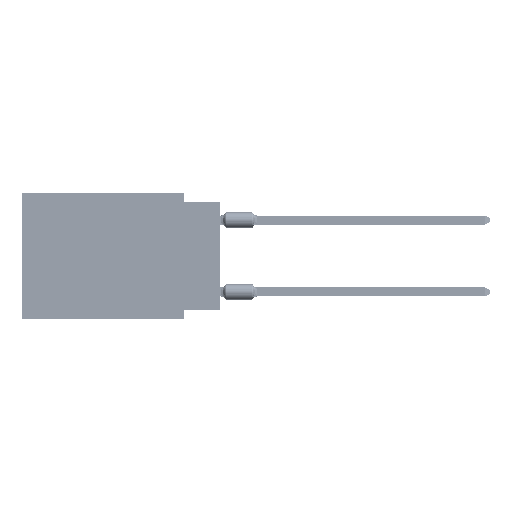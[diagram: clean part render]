
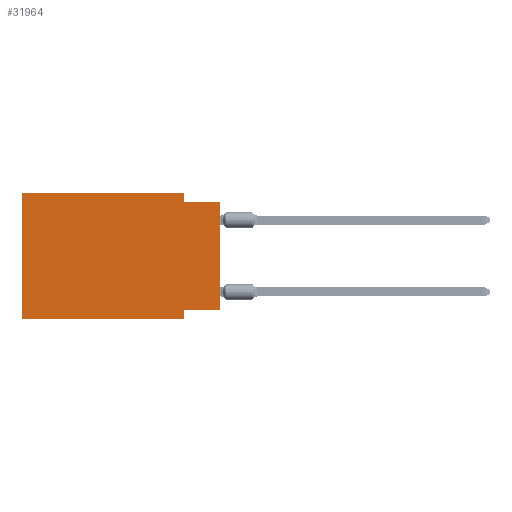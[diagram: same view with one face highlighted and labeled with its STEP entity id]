
A CAD part, left-side view. The second image highlights one B-rep face of the part: STEP entity #31964.
In plain terms, the highlighted planar face has unit normal (-1, 0, 0).
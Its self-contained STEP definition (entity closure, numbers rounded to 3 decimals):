
#1317 = ORIENTED_EDGE ( 'NONE', *, *, #56635, .F. ) ;
#4426 = EDGE_CURVE ( 'NONE', #86143, #73094, #27593, .T. ) ;
#5830 = CARTESIAN_POINT ( 'NONE',  ( 0., 13.97, -8.89 ) ) ;
#7325 = VECTOR ( 'NONE', #56872, 1000. ) ;
#10690 = VERTEX_POINT ( 'NONE', #80825 ) ;
#12012 = ORIENTED_EDGE ( 'NONE', *, *, #41503, .T. ) ;
#13321 = CARTESIAN_POINT ( 'NONE',  ( 0., 0., -8.255 ) ) ;
#13442 = DIRECTION ( 'NONE',  ( 0., 0., -1. ) ) ;
#14587 = CARTESIAN_POINT ( 'NONE',  ( 0., 13.97, 0. ) ) ;
#18264 = EDGE_LOOP ( 'NONE', ( #12012, #1317, #19668, #59747, #22438, #51683, #84203, #18834 ) ) ;
#18834 = ORIENTED_EDGE ( 'NONE', *, *, #32896, .F. ) ;
#19668 = ORIENTED_EDGE ( 'NONE', *, *, #21820, .F. ) ;
#20445 = CARTESIAN_POINT ( 'NONE',  ( 0., 13.97, 0. ) ) ;
#21051 = VERTEX_POINT ( 'NONE', #76989 ) ;
#21820 = EDGE_CURVE ( 'NONE', #10690, #73108, #37596, .T. ) ;
#22028 = DIRECTION ( 'NONE',  ( 0., 0., 1. ) ) ;
#22196 = CARTESIAN_POINT ( 'NONE',  ( 0., 2.54, 0. ) ) ;
#22438 = ORIENTED_EDGE ( 'NONE', *, *, #80332, .F. ) ;
#23707 = CARTESIAN_POINT ( 'NONE',  ( 0., 13.97, -8.89 ) ) ;
#24312 = AXIS2_PLACEMENT_3D ( 'NONE', #20445, #77865, #13442 ) ;
#27593 = LINE ( 'NONE', #49036, #48803 ) ;
#28555 = CARTESIAN_POINT ( 'NONE',  ( 0., 0., 0. ) ) ;
#29881 = EDGE_CURVE ( 'NONE', #78756, #73094, #51234, .T. ) ;
#31964 = ADVANCED_FACE ( 'NONE', ( #56815 ), #84426, .F. ) ;
#32896 = EDGE_CURVE ( 'NONE', #46298, #86143, #88183, .T. ) ;
#35428 = LINE ( 'NONE', #63883, #7325 ) ;
#37596 = LINE ( 'NONE', #22196, #53891 ) ;
#41503 = EDGE_CURVE ( 'NONE', #46298, #58428, #55608, .T. ) ;
#43671 = DIRECTION ( 'NONE',  ( 0., 0., -1. ) ) ;
#46298 = VERTEX_POINT ( 'NONE', #13321 ) ;
#48803 = VECTOR ( 'NONE', #76147, 1000. ) ;
#49036 = CARTESIAN_POINT ( 'NONE',  ( 0., 2.54, -8.89 ) ) ;
#51234 = LINE ( 'NONE', #23707, #55578 ) ;
#51683 = ORIENTED_EDGE ( 'NONE', *, *, #29881, .T. ) ;
#53869 = LINE ( 'NONE', #67877, #61285 ) ;
#53891 = VECTOR ( 'NONE', #43671, 1000. ) ;
#55578 = VECTOR ( 'NONE', #58256, 1000. ) ;
#55608 = LINE ( 'NONE', #28555, #79543 ) ;
#56635 = EDGE_CURVE ( 'NONE', #73108, #58428, #35428, .T. ) ;
#56815 = FACE_OUTER_BOUND ( 'NONE', #18264, .T. ) ;
#56872 = DIRECTION ( 'NONE',  ( 0., -1., 0. ) ) ;
#58256 = DIRECTION ( 'NONE',  ( 0., -1., 0. ) ) ;
#58428 = VERTEX_POINT ( 'NONE', #72510 ) ;
#59747 = ORIENTED_EDGE ( 'NONE', *, *, #66436, .F. ) ;
#60871 = DIRECTION ( 'NONE',  ( 0., -1., 0. ) ) ;
#61285 = VECTOR ( 'NONE', #60871, 1000. ) ;
#61506 = DIRECTION ( 'NONE',  ( 0., 1., 0. ) ) ;
#63883 = CARTESIAN_POINT ( 'NONE',  ( 0., 0., -0.635 ) ) ;
#64071 = LINE ( 'NONE', #14587, #67506 ) ;
#64471 = DIRECTION ( 'NONE',  ( 0., 0., 1. ) ) ;
#66436 = EDGE_CURVE ( 'NONE', #21051, #10690, #53869, .T. ) ;
#67267 = CARTESIAN_POINT ( 'NONE',  ( 0., 2.54, -8.255 ) ) ;
#67506 = VECTOR ( 'NONE', #22028, 1000. ) ;
#67877 = CARTESIAN_POINT ( 'NONE',  ( 0., 13.97, 0. ) ) ;
#72510 = CARTESIAN_POINT ( 'NONE',  ( 0., 0., -0.635 ) ) ;
#73094 = VERTEX_POINT ( 'NONE', #79990 ) ;
#73108 = VERTEX_POINT ( 'NONE', #80455 ) ;
#76147 = DIRECTION ( 'NONE',  ( 0., 0., -1. ) ) ;
#76989 = CARTESIAN_POINT ( 'NONE',  ( 0., 13.97, 0. ) ) ;
#77865 = DIRECTION ( 'NONE',  ( 1., 0., 0. ) ) ;
#78756 = VERTEX_POINT ( 'NONE', #5830 ) ;
#79543 = VECTOR ( 'NONE', #64471, 1000. ) ;
#79990 = CARTESIAN_POINT ( 'NONE',  ( 0., 2.54, -8.89 ) ) ;
#80332 = EDGE_CURVE ( 'NONE', #78756, #21051, #64071, .T. ) ;
#80455 = CARTESIAN_POINT ( 'NONE',  ( 0., 2.54, -0.635 ) ) ;
#80825 = CARTESIAN_POINT ( 'NONE',  ( 0., 2.54, 0. ) ) ;
#81623 = CARTESIAN_POINT ( 'NONE',  ( 0., 0., -8.255 ) ) ;
#84203 = ORIENTED_EDGE ( 'NONE', *, *, #4426, .F. ) ;
#84426 = PLANE ( 'NONE',  #24312 ) ;
#85543 = VECTOR ( 'NONE', #61506, 1000. ) ;
#86143 = VERTEX_POINT ( 'NONE', #67267 ) ;
#88183 = LINE ( 'NONE', #81623, #85543 ) ;
